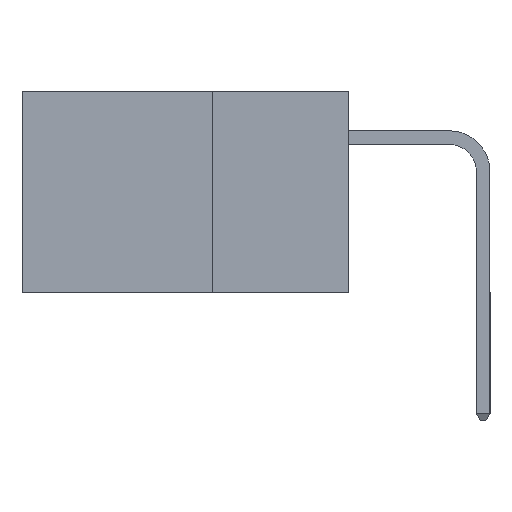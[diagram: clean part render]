
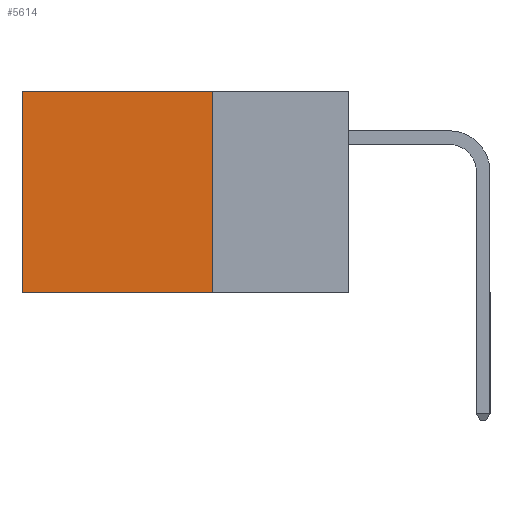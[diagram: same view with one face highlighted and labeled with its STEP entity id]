
A CAD part, left-side view. The second image highlights one B-rep face of the part: STEP entity #5614.
In plain terms, the highlighted planar face has unit normal (-1, 0, 0).
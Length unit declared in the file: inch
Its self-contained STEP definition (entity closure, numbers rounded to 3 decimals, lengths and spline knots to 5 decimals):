
#191 = EDGE_LOOP ( 'NONE', ( #1470, #1474, #1729, #1912 ) ) ;
#263 = FACE_OUTER_BOUND ( 'NONE', #191, .T. ) ;
#902 = VERTEX_POINT ( 'NONE', #6555 ) ;
#1449 = DIRECTION ( 'NONE',  ( 0., 1., 0. ) ) ;
#1470 = ORIENTED_EDGE ( 'NONE', *, *, #3825, .T. ) ;
#1474 = ORIENTED_EDGE ( 'NONE', *, *, #8436, .F. ) ;
#1729 = ORIENTED_EDGE ( 'NONE', *, *, #10539, .F. ) ;
#1804 = LINE ( 'NONE', #4463, #11147 ) ;
#1912 = ORIENTED_EDGE ( 'NONE', *, *, #11120, .T. ) ;
#3471 = DIRECTION ( 'NONE',  ( 0., 0., -1. ) ) ;
#3825 = EDGE_CURVE ( 'NONE', #10782, #6865, #11880, .T. ) ;
#4463 = CARTESIAN_POINT ( 'NONE',  ( 0.2875, 0.25, 0. ) ) ;
#5324 = CARTESIAN_POINT ( 'NONE',  ( 0.2875, 0.25, 0. ) ) ;
#5446 = CARTESIAN_POINT ( 'NONE',  ( 0.2875, 0.6, 0. ) ) ;
#5614 = ADVANCED_FACE ( 'NONE', ( #263 ), #9779, .F. ) ;
#5829 = CARTESIAN_POINT ( 'NONE',  ( 0.2875, 0.6, 0. ) ) ;
#6313 = DIRECTION ( 'NONE',  ( 0., 0., -1. ) ) ;
#6555 = CARTESIAN_POINT ( 'NONE',  ( 0.2875, 0.25, -0.37 ) ) ;
#6865 = VERTEX_POINT ( 'NONE', #9635 ) ;
#7077 = AXIS2_PLACEMENT_3D ( 'NONE', #5324, #11312, #6313 ) ;
#7310 = CARTESIAN_POINT ( 'NONE',  ( 0.2875, 0.25, 0. ) ) ;
#7317 = VERTEX_POINT ( 'NONE', #8550 ) ;
#7359 = DIRECTION ( 'NONE',  ( 0., 0., -1. ) ) ;
#7918 = VECTOR ( 'NONE', #9434, 39.37008 ) ;
#8436 = EDGE_CURVE ( 'NONE', #902, #6865, #10383, .T. ) ;
#8550 = CARTESIAN_POINT ( 'NONE',  ( 0.2875, 0.25, 0. ) ) ;
#8562 = CARTESIAN_POINT ( 'NONE',  ( 0.2875, 0.25, -0.37 ) ) ;
#9434 = DIRECTION ( 'NONE',  ( 0., 1., 0. ) ) ;
#9591 = VECTOR ( 'NONE', #1449, 39.37008 ) ;
#9635 = CARTESIAN_POINT ( 'NONE',  ( 0.2875, 0.6, -0.37 ) ) ;
#9779 = PLANE ( 'NONE',  #7077 ) ;
#9837 = VECTOR ( 'NONE', #7359, 39.37008 ) ;
#10383 = LINE ( 'NONE', #8562, #7918 ) ;
#10539 = EDGE_CURVE ( 'NONE', #7317, #902, #1804, .T. ) ;
#10782 = VERTEX_POINT ( 'NONE', #5829 ) ;
#11120 = EDGE_CURVE ( 'NONE', #7317, #10782, #11401, .T. ) ;
#11147 = VECTOR ( 'NONE', #3471, 39.37008 ) ;
#11312 = DIRECTION ( 'NONE',  ( 1., 0., 0. ) ) ;
#11401 = LINE ( 'NONE', #7310, #9591 ) ;
#11880 = LINE ( 'NONE', #5446, #9837 ) ;
